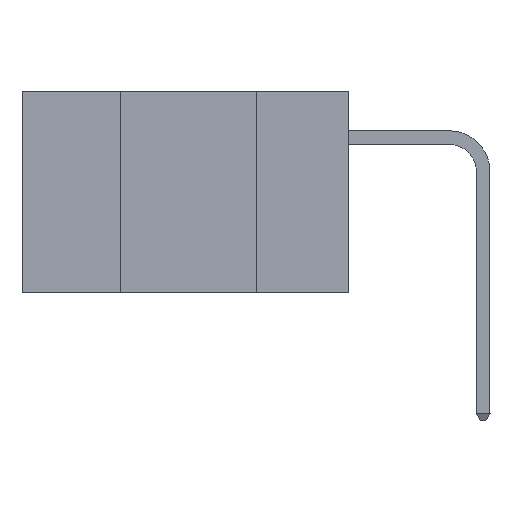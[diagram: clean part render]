
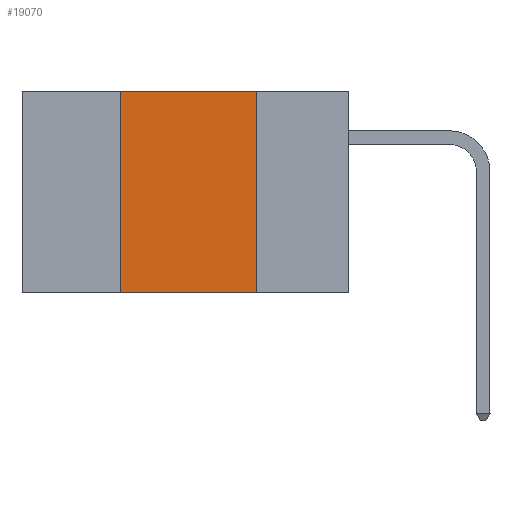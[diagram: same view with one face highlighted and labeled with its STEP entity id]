
A CAD part, left-side view. The second image highlights one B-rep face of the part: STEP entity #19070.
In plain terms, the highlighted planar face has unit normal (-1, 0, 0).
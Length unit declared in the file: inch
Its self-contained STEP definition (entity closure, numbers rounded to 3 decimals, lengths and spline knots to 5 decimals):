
#992 = DIRECTION ( 'NONE',  ( 1., 0., 0. ) ) ;
#1528 = LINE ( 'NONE', #25595, #30990 ) ;
#2524 = VERTEX_POINT ( 'NONE', #14662 ) ;
#3722 = VERTEX_POINT ( 'NONE', #26333 ) ;
#7216 = CARTESIAN_POINT ( 'NONE',  ( 0., 0.6, 0. ) ) ;
#7316 = VECTOR ( 'NONE', #25377, 39.37008 ) ;
#7511 = CARTESIAN_POINT ( 'NONE',  ( 0., 0.6, -0.37 ) ) ;
#8285 = VERTEX_POINT ( 'NONE', #36171 ) ;
#9173 = EDGE_CURVE ( 'NONE', #3722, #18755, #14908, .T. ) ;
#9856 = CARTESIAN_POINT ( 'NONE',  ( 0., 0.42, 0. ) ) ;
#11586 = VECTOR ( 'NONE', #20557, 39.37008 ) ;
#13003 = VECTOR ( 'NONE', #21705, 39.37008 ) ;
#13570 = ORIENTED_EDGE ( 'NONE', *, *, #25181, .F. ) ;
#14021 = ORIENTED_EDGE ( 'NONE', *, *, #9173, .F. ) ;
#14662 = CARTESIAN_POINT ( 'NONE',  ( 0., 0.42, -0.37 ) ) ;
#14908 = LINE ( 'NONE', #36109, #11586 ) ;
#17324 = ORIENTED_EDGE ( 'NONE', *, *, #26795, .T. ) ;
#18755 = VERTEX_POINT ( 'NONE', #22019 ) ;
#19060 = PLANE ( 'NONE',  #28793 ) ;
#19070 = ADVANCED_FACE ( 'NONE', ( #33857 ), #19060, .F. ) ;
#20557 = DIRECTION ( 'NONE',  ( 0., -1., 0. ) ) ;
#21705 = DIRECTION ( 'NONE',  ( 0., 0., 1. ) ) ;
#22019 = CARTESIAN_POINT ( 'NONE',  ( 0., 0.17, 0. ) ) ;
#22077 = LINE ( 'NONE', #7511, #7316 ) ;
#25181 = EDGE_CURVE ( 'NONE', #18755, #8285, #1528, .T. ) ;
#25377 = DIRECTION ( 'NONE',  ( 0., -1., 0. ) ) ;
#25595 = CARTESIAN_POINT ( 'NONE',  ( 0., 0.17, 0. ) ) ;
#26333 = CARTESIAN_POINT ( 'NONE',  ( 0., 0.42, 0. ) ) ;
#26795 = EDGE_CURVE ( 'NONE', #2524, #8285, #22077, .T. ) ;
#28793 = AXIS2_PLACEMENT_3D ( 'NONE', #7216, #992, #30736 ) ;
#28900 = DIRECTION ( 'NONE',  ( 0., 0., -1. ) ) ;
#29177 = EDGE_CURVE ( 'NONE', #2524, #3722, #30658, .T. ) ;
#29604 = EDGE_LOOP ( 'NONE', ( #13570, #14021, #38172, #17324 ) ) ;
#30658 = LINE ( 'NONE', #9856, #13003 ) ;
#30736 = DIRECTION ( 'NONE',  ( 0., 0., -1. ) ) ;
#30990 = VECTOR ( 'NONE', #28900, 39.37008 ) ;
#33857 = FACE_OUTER_BOUND ( 'NONE', #29604, .T. ) ;
#36109 = CARTESIAN_POINT ( 'NONE',  ( 0., 0.6, 0. ) ) ;
#36171 = CARTESIAN_POINT ( 'NONE',  ( 0., 0.17, -0.37 ) ) ;
#38172 = ORIENTED_EDGE ( 'NONE', *, *, #29177, .F. ) ;
